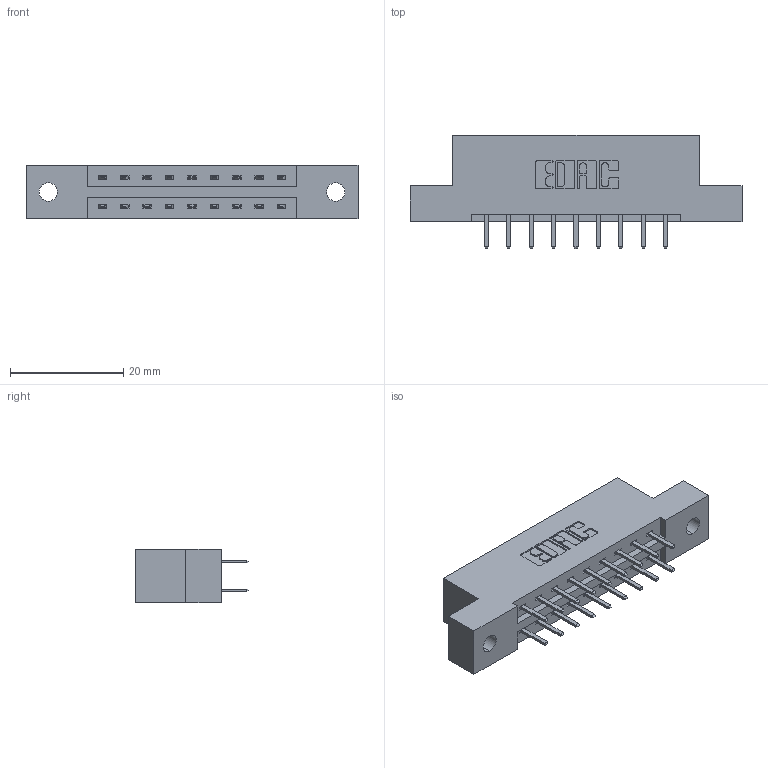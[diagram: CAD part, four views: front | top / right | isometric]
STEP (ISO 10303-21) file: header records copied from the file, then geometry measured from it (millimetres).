
FILE_DESCRIPTION (( 'STEP AP203' ), '1' );
FILE_NAME ('387-018-520-202.STEP', '2019-10-16T00:22:58', ( '' ), ( '' ), 'SwSTEP 2.0', 'SolidWorks 2016', '' );
FILE_SCHEMA (( 'CONFIG_CONTROL_DESIGN' ));
Length unit declared in the file: inch
Products named in the file (3): 337 Part_Flush Mounting Lugs - 0.128 Dia; 387-018-520-202; 345-292-001_345-293-120
Assembly tree (19 placements, depth 2):
  387-018-520-202
    337 Part_Flush Mounting Lugs - 0.128 Dia
    345-292-001_345-293-120  x18
Bounding box: 58.67 x 20.02 x 9.4 mm (x, y, z)
Volume: 5699.7 mm3; surface area: 5827.7 mm2
Topology: 19 solids, 19 shells, 1158 faces, 3353 edges, 2186 vertices
Faces by surface type: plane 790, cylinder 368
Entity records: 11363 total; most frequent: CARTESIAN_POINT 1954, ORIENTED_EDGE 1878, DIRECTION 1711, EDGE_CURVE 939, LINE 807, VECTOR 807, VERTEX_POINT 622, AXIS2_PLACEMENT_3D 452
